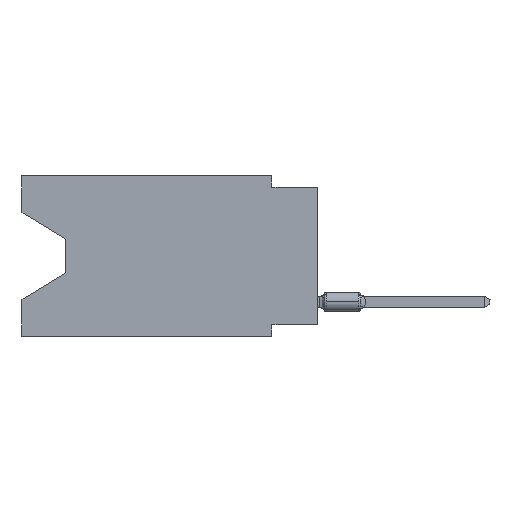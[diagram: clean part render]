
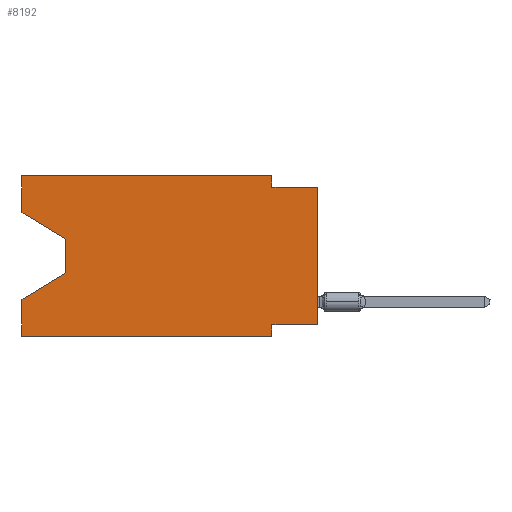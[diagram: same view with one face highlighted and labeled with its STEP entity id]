
A CAD part, left-side view. The second image highlights one B-rep face of the part: STEP entity #8192.
In plain terms, the highlighted planar face has unit normal (-1, 0, 0).
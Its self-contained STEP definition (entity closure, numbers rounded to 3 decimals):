
#1437 = CARTESIAN_POINT ( 'NONE',  ( 0., 2.54, -8.89 ) ) ;
#8165 = ORIENTED_EDGE ( 'NONE', *, *, #23473, .T. ) ;
#8192 = ADVANCED_FACE ( 'NONE', ( #10361 ), #69472, .F. ) ;
#8200 = VECTOR ( 'NONE', #69456, 1000. ) ;
#9019 = LINE ( 'NONE', #83480, #61479 ) ;
#9271 = ORIENTED_EDGE ( 'NONE', *, *, #55312, .F. ) ;
#9870 = CARTESIAN_POINT ( 'NONE',  ( 0., 16.383, 0. ) ) ;
#10020 = CARTESIAN_POINT ( 'NONE',  ( 0., 2.54, -0.635 ) ) ;
#10361 = FACE_OUTER_BOUND ( 'NONE', #24536, .T. ) ;
#10898 = VERTEX_POINT ( 'NONE', #74569 ) ;
#13535 = VECTOR ( 'NONE', #28663, 1000. ) ;
#13940 = LINE ( 'NONE', #23364, #89093 ) ;
#14534 = ORIENTED_EDGE ( 'NONE', *, *, #66813, .F. ) ;
#15123 = LINE ( 'NONE', #23556, #91730 ) ;
#15382 = EDGE_CURVE ( 'NONE', #38219, #56212, #15123, .T. ) ;
#15400 = DIRECTION ( 'NONE',  ( 0., -1., 0. ) ) ;
#15750 = DIRECTION ( 'NONE',  ( 0., 1., 0. ) ) ;
#17330 = VERTEX_POINT ( 'NONE', #79926 ) ;
#18310 = VECTOR ( 'NONE', #63333, 1000. ) ;
#18565 = VECTOR ( 'NONE', #15750, 1000. ) ;
#19836 = CARTESIAN_POINT ( 'NONE',  ( 0., 16.383, 0. ) ) ;
#20798 = CARTESIAN_POINT ( 'NONE',  ( 0., 2.54, 0. ) ) ;
#21644 = DIRECTION ( 'NONE',  ( 0., 0., -1. ) ) ;
#23364 = CARTESIAN_POINT ( 'NONE',  ( 0., 0., 0. ) ) ;
#23473 = EDGE_CURVE ( 'NONE', #52740, #27319, #94575, .T. ) ;
#23556 = CARTESIAN_POINT ( 'NONE',  ( 0., 2.54, 0. ) ) ;
#24536 = EDGE_LOOP ( 'NONE', ( #8165, #88650, #65821, #79531, #95533, #97973, #73041, #69710, #14534, #54588, #72447, #9271 ) ) ;
#25487 = VERTEX_POINT ( 'NONE', #67082 ) ;
#27319 = VERTEX_POINT ( 'NONE', #34649 ) ;
#28663 = DIRECTION ( 'NONE',  ( 0., -1., 0. ) ) ;
#29704 = CARTESIAN_POINT ( 'NONE',  ( 0., 16.383, -2.038 ) ) ;
#30150 = LINE ( 'NONE', #66888, #13535 ) ;
#31309 = DIRECTION ( 'NONE',  ( 0., 0., 1. ) ) ;
#32687 = VERTEX_POINT ( 'NONE', #96365 ) ;
#33040 = LINE ( 'NONE', #47467, #89080 ) ;
#33353 = VECTOR ( 'NONE', #21644, 1000. ) ;
#34649 = CARTESIAN_POINT ( 'NONE',  ( 0., 13.97, -3.505 ) ) ;
#37232 = EDGE_CURVE ( 'NONE', #17330, #25487, #55407, .T. ) ;
#37329 = DIRECTION ( 'NONE',  ( 0., 0.855, -0.519 ) ) ;
#38219 = VERTEX_POINT ( 'NONE', #20798 ) ;
#39147 = EDGE_CURVE ( 'NONE', #67028, #25487, #9019, .T. ) ;
#40664 = DIRECTION ( 'NONE',  ( 0., 0., -1. ) ) ;
#41387 = VECTOR ( 'NONE', #55063, 1000. ) ;
#42480 = CARTESIAN_POINT ( 'NONE',  ( 0., 16.383, -2.038 ) ) ;
#42521 = EDGE_CURVE ( 'NONE', #53118, #10898, #51600, .T. ) ;
#42746 = LINE ( 'NONE', #96313, #61293 ) ;
#45433 = DIRECTION ( 'NONE',  ( 0., 0., -1. ) ) ;
#47467 = CARTESIAN_POINT ( 'NONE',  ( 0., 16.383, -8.89 ) ) ;
#48928 = CARTESIAN_POINT ( 'NONE',  ( 0., 16.383, 0. ) ) ;
#49080 = EDGE_CURVE ( 'NONE', #85777, #32687, #13940, .T. ) ;
#50216 = AXIS2_PLACEMENT_3D ( 'NONE', #9870, #54118, #40664 ) ;
#51600 = LINE ( 'NONE', #1437, #41387 ) ;
#52446 = LINE ( 'NONE', #94759, #33353 ) ;
#52740 = VERTEX_POINT ( 'NONE', #29704 ) ;
#52901 = VECTOR ( 'NONE', #15400, 1000. ) ;
#53118 = VERTEX_POINT ( 'NONE', #83680 ) ;
#54118 = DIRECTION ( 'NONE',  ( 1., 0., 0. ) ) ;
#54588 = ORIENTED_EDGE ( 'NONE', *, *, #15382, .F. ) ;
#55063 = DIRECTION ( 'NONE',  ( 0., 0., -1. ) ) ;
#55312 = EDGE_CURVE ( 'NONE', #52740, #78142, #42746, .T. ) ;
#55407 = LINE ( 'NONE', #48928, #18310 ) ;
#56212 = VERTEX_POINT ( 'NONE', #10020 ) ;
#58382 = CARTESIAN_POINT ( 'NONE',  ( 0., 13.97, -5.385 ) ) ;
#61293 = VECTOR ( 'NONE', #81912, 1000. ) ;
#61368 = EDGE_CURVE ( 'NONE', #17330, #10898, #33040, .T. ) ;
#61479 = VECTOR ( 'NONE', #37329, 1000. ) ;
#63307 = EDGE_CURVE ( 'NONE', #78142, #38219, #83396, .T. ) ;
#63333 = DIRECTION ( 'NONE',  ( 0., 0., 1. ) ) ;
#64276 = CARTESIAN_POINT ( 'NONE',  ( 0., 0., -8.255 ) ) ;
#65821 = ORIENTED_EDGE ( 'NONE', *, *, #39147, .T. ) ;
#66813 = EDGE_CURVE ( 'NONE', #56212, #32687, #30150, .T. ) ;
#66888 = CARTESIAN_POINT ( 'NONE',  ( 0., 0., -0.635 ) ) ;
#67028 = VERTEX_POINT ( 'NONE', #58382 ) ;
#67082 = CARTESIAN_POINT ( 'NONE',  ( 0., 16.383, -6.852 ) ) ;
#69456 = DIRECTION ( 'NONE',  ( 0., -0.855, -0.519 ) ) ;
#69472 = PLANE ( 'NONE',  #50216 ) ;
#69487 = CARTESIAN_POINT ( 'NONE',  ( 0., 16.383, 0. ) ) ;
#69710 = ORIENTED_EDGE ( 'NONE', *, *, #49080, .T. ) ;
#69773 = DIRECTION ( 'NONE',  ( 0., -1., 0. ) ) ;
#71657 = LINE ( 'NONE', #79576, #18565 ) ;
#72447 = ORIENTED_EDGE ( 'NONE', *, *, #63307, .F. ) ;
#73041 = ORIENTED_EDGE ( 'NONE', *, *, #91317, .F. ) ;
#74569 = CARTESIAN_POINT ( 'NONE',  ( 0., 2.54, -8.89 ) ) ;
#78142 = VERTEX_POINT ( 'NONE', #19836 ) ;
#79531 = ORIENTED_EDGE ( 'NONE', *, *, #37232, .F. ) ;
#79576 = CARTESIAN_POINT ( 'NONE',  ( 0., 0., -8.255 ) ) ;
#79926 = CARTESIAN_POINT ( 'NONE',  ( 0., 16.383, -8.89 ) ) ;
#81912 = DIRECTION ( 'NONE',  ( 0., 0., 1. ) ) ;
#83396 = LINE ( 'NONE', #69487, #52901 ) ;
#83480 = CARTESIAN_POINT ( 'NONE',  ( 0., 13.97, -5.385 ) ) ;
#83680 = CARTESIAN_POINT ( 'NONE',  ( 0., 2.54, -8.255 ) ) ;
#85777 = VERTEX_POINT ( 'NONE', #64276 ) ;
#88650 = ORIENTED_EDGE ( 'NONE', *, *, #94966, .T. ) ;
#89080 = VECTOR ( 'NONE', #69773, 1000. ) ;
#89093 = VECTOR ( 'NONE', #31309, 1000. ) ;
#91317 = EDGE_CURVE ( 'NONE', #85777, #53118, #71657, .T. ) ;
#91730 = VECTOR ( 'NONE', #45433, 1000. ) ;
#94575 = LINE ( 'NONE', #42480, #8200 ) ;
#94759 = CARTESIAN_POINT ( 'NONE',  ( 0., 13.97, -3.505 ) ) ;
#94966 = EDGE_CURVE ( 'NONE', #27319, #67028, #52446, .T. ) ;
#95533 = ORIENTED_EDGE ( 'NONE', *, *, #61368, .T. ) ;
#96313 = CARTESIAN_POINT ( 'NONE',  ( 0., 16.383, 0. ) ) ;
#96365 = CARTESIAN_POINT ( 'NONE',  ( 0., 0., -0.635 ) ) ;
#97973 = ORIENTED_EDGE ( 'NONE', *, *, #42521, .F. ) ;
